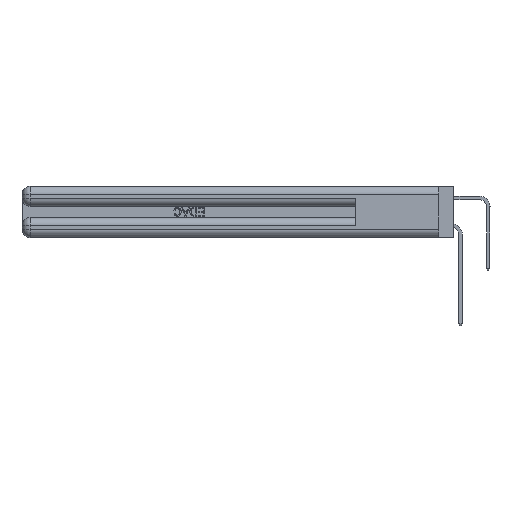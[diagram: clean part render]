
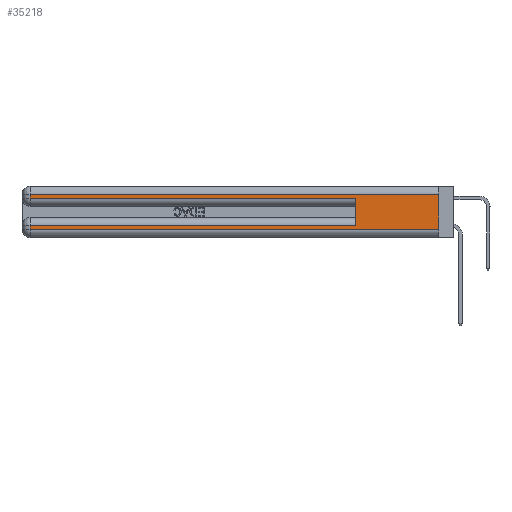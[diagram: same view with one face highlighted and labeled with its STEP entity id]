
A CAD part, left-side view. The second image highlights one B-rep face of the part: STEP entity #35218.
In plain terms, the highlighted planar face has unit normal (-1, 0, 0).
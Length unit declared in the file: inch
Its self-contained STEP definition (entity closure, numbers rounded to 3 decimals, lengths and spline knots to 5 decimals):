
#17 = DIRECTION ( 'NONE',  ( 0., 0., -1. ) ) ;
#167 = ORIENTED_EDGE ( 'NONE', *, *, #41132, .T. ) ;
#430 = ORIENTED_EDGE ( 'NONE', *, *, #27897, .F. ) ;
#578 = VECTOR ( 'NONE', #47433, 39.37008 ) ;
#961 = VECTOR ( 'NONE', #23020, 39.37008 ) ;
#1434 = DIRECTION ( 'NONE',  ( 0., 0., -1. ) ) ;
#1503 = ORIENTED_EDGE ( 'NONE', *, *, #21060, .T. ) ;
#1524 = EDGE_CURVE ( 'NONE', #41081, #36736, #29479, .T. ) ;
#1766 = CARTESIAN_POINT ( 'NONE',  ( 0., 2.94, 0.085 ) ) ;
#1810 = CARTESIAN_POINT ( 'NONE',  ( 0., 2.94, 0.31 ) ) ;
#1934 = CARTESIAN_POINT ( 'NONE',  ( 0., 0., 0.085 ) ) ;
#2812 = VERTEX_POINT ( 'NONE', #19103 ) ;
#2932 = ORIENTED_EDGE ( 'NONE', *, *, #40781, .T. ) ;
#3708 = LINE ( 'NONE', #1934, #22431 ) ;
#8881 = CARTESIAN_POINT ( 'NONE',  ( 0., 0., 0.37 ) ) ;
#8920 = EDGE_CURVE ( 'NONE', #36736, #40903, #26119, .T. ) ;
#9719 = ORIENTED_EDGE ( 'NONE', *, *, #8920, .T. ) ;
#10845 = ORIENTED_EDGE ( 'NONE', *, *, #20647, .T. ) ;
#11323 = FACE_OUTER_BOUND ( 'NONE', #46731, .T. ) ;
#12034 = CARTESIAN_POINT ( 'NONE',  ( 0., 0., 0.06 ) ) ;
#12201 = LINE ( 'NONE', #15561, #961 ) ;
#12642 = DIRECTION ( 'NONE',  ( 0., 0., -1. ) ) ;
#14909 = AXIS2_PLACEMENT_3D ( 'NONE', #8881, #23890, #1434 ) ;
#15060 = CARTESIAN_POINT ( 'NONE',  ( 0., 2.94, 0.37 ) ) ;
#15561 = CARTESIAN_POINT ( 'NONE',  ( 0., 0., 0.37 ) ) ;
#16227 = VECTOR ( 'NONE', #31217, 39.37008 ) ;
#16940 = EDGE_CURVE ( 'NONE', #2812, #40903, #12201, .T. ) ;
#17689 = ORIENTED_EDGE ( 'NONE', *, *, #16940, .F. ) ;
#19103 = CARTESIAN_POINT ( 'NONE',  ( 0., 0., 0.31 ) ) ;
#19413 = LINE ( 'NONE', #43683, #578 ) ;
#20647 = EDGE_CURVE ( 'NONE', #23640, #40184, #19413, .T. ) ;
#21060 = EDGE_CURVE ( 'NONE', #2812, #38268, #32725, .T. ) ;
#22431 = VECTOR ( 'NONE', #31854, 39.37008 ) ;
#22848 = VECTOR ( 'NONE', #31294, 39.37008 ) ;
#22867 = ORIENTED_EDGE ( 'NONE', *, *, #1524, .T. ) ;
#23020 = DIRECTION ( 'NONE',  ( 0., 0., -1. ) ) ;
#23626 = CARTESIAN_POINT ( 'NONE',  ( 0., 2.94, 0.285 ) ) ;
#23640 = VERTEX_POINT ( 'NONE', #23626 ) ;
#23821 = CARTESIAN_POINT ( 'NONE',  ( 0., 0., 0.31 ) ) ;
#23890 = DIRECTION ( 'NONE',  ( 1., 0., 0. ) ) ;
#26077 = CARTESIAN_POINT ( 'NONE',  ( 0., 0.6, 0.145 ) ) ;
#26119 = LINE ( 'NONE', #27489, #16227 ) ;
#27489 = CARTESIAN_POINT ( 'NONE',  ( 0., 0., 0.06 ) ) ;
#27728 = VECTOR ( 'NONE', #12642, 39.37008 ) ;
#27897 = EDGE_CURVE ( 'NONE', #41317, #40184, #45251, .T. ) ;
#28890 = LINE ( 'NONE', #45979, #27728 ) ;
#29479 = LINE ( 'NONE', #15060, #45766 ) ;
#29800 = DIRECTION ( 'NONE',  ( 0., 0., 1. ) ) ;
#31217 = DIRECTION ( 'NONE',  ( 0., -1., 0. ) ) ;
#31294 = DIRECTION ( 'NONE',  ( 0., 1., 0. ) ) ;
#31378 = CARTESIAN_POINT ( 'NONE',  ( 0., 0.6, 0.085 ) ) ;
#31854 = DIRECTION ( 'NONE',  ( 0., 1., 0. ) ) ;
#32725 = LINE ( 'NONE', #23821, #22848 ) ;
#33798 = CARTESIAN_POINT ( 'NONE',  ( 0., 2.94, 0.06 ) ) ;
#35218 = ADVANCED_FACE ( 'NONE', ( #11323 ), #42419, .F. ) ;
#35341 = VECTOR ( 'NONE', #29800, 39.37008 ) ;
#35431 = CARTESIAN_POINT ( 'NONE',  ( 0., 0.6, 0.285 ) ) ;
#36736 = VERTEX_POINT ( 'NONE', #33798 ) ;
#38268 = VERTEX_POINT ( 'NONE', #1810 ) ;
#40184 = VERTEX_POINT ( 'NONE', #35431 ) ;
#40781 = EDGE_CURVE ( 'NONE', #38268, #23640, #28890, .T. ) ;
#40903 = VERTEX_POINT ( 'NONE', #12034 ) ;
#41081 = VERTEX_POINT ( 'NONE', #1766 ) ;
#41132 = EDGE_CURVE ( 'NONE', #41317, #41081, #3708, .T. ) ;
#41317 = VERTEX_POINT ( 'NONE', #31378 ) ;
#42419 = PLANE ( 'NONE',  #14909 ) ;
#43683 = CARTESIAN_POINT ( 'NONE',  ( 0., 0., 0.285 ) ) ;
#45251 = LINE ( 'NONE', #26077, #35341 ) ;
#45766 = VECTOR ( 'NONE', #17, 39.37008 ) ;
#45979 = CARTESIAN_POINT ( 'NONE',  ( 0., 2.94, 0.37 ) ) ;
#46731 = EDGE_LOOP ( 'NONE', ( #17689, #1503, #2932, #10845, #430, #167, #22867, #9719 ) ) ;
#47433 = DIRECTION ( 'NONE',  ( 0., -1., 0. ) ) ;
